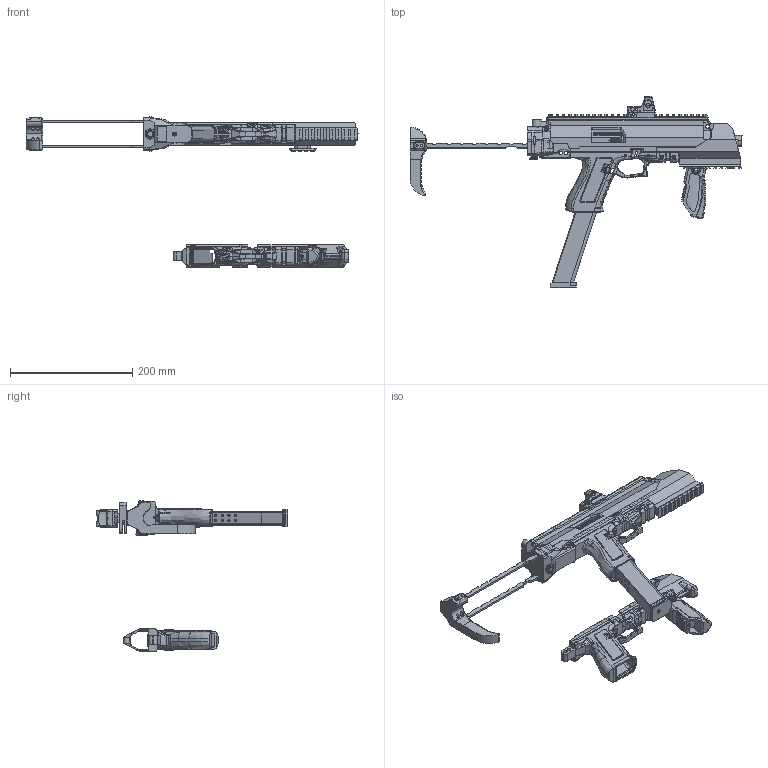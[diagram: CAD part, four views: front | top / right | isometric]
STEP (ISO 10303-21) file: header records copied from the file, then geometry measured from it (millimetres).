
FILE_DESCRIPTION(/* description */ (''),/* implementation_level */ '2;1');
FILE_NAME(/* name */ 'Unseenkiller Remix - MP17.step',/* time_stamp */ '2023-01-13T11:15:07-05:00',/* author */ (''),/* organization */ (''),/* preprocessor_version */ 'ST-DEVELOPER v19.2',/* originating_system */ 'Autodesk Translation Framework v11.17.0.187',/* authorisation */ '');
FILE_SCHEMA (('AUTOMOTIVE_DESIGN { 1 0 10303 214 3 1 1 }'));
Products named in the file (9): Unseenkiller Remix - MP17; Trijicon RMR Optic (3); Right Button (3); Glass (3); Mount Clip (3); Left Button (3); Optic Housing (1) (3); RMR Footprint Adapter Plate (1) (3); Danny Meatball - XL 9mm Mag (1)
Assembly tree (8 placements, depth 3):
  Unseenkiller Remix - MP17
    Trijicon RMR Optic (3)
      Right Button (3)
      Glass (3)
      Mount Clip (3)
      Left Button (3)
      Optic Housing (1) (3)
      RMR Footprint Adapter Plate (1) (3)
    Danny Meatball - XL 9mm Mag (1)
Bounding box: 543.17 x 312.98 x 246.92 mm (x, y, z)
Volume: 885184.4 mm3; surface area: 427029.8 mm2
Topology: 27 solids, 54 shells, 5670 faces, 15735 edges, 10069 vertices
Faces by surface type: plane 2464, bspline 1511, cylinder 1226, torus 280, sphere 120, cone 69
Full cylindrical faces by diameter (mm): 1.27 x2, 1.75 x1, 2 x1, 3 x24, 3.048 x1, 3.1 x4, 3.2 x2, 3.242 x6, 3.5 x12, 3.7 x1, 4 x8, 4.064 x1, 4.15 x2, 4.2 x3, 4.572 x1, 5 x6, 5.035 x27, 5.105 x1, 5.156 x3, 5.5 x1, 6 x17, 6.045 x1, 6.147 x27, 7.2 x2, 7.366 x1, 7.62 x1, 7.7 x4, 8.001 x1, 8.82 x1, 8.858 x1
Entity records: 413262 total; most frequent: CARTESIAN_POINT 276962, ORIENTED_EDGE 31294, DIRECTION 23943, EDGE_CURVE 15647, VERTEX_POINT 10069, LINE 8567, VECTOR 8567, AXIS2_PLACEMENT_3D 7688
